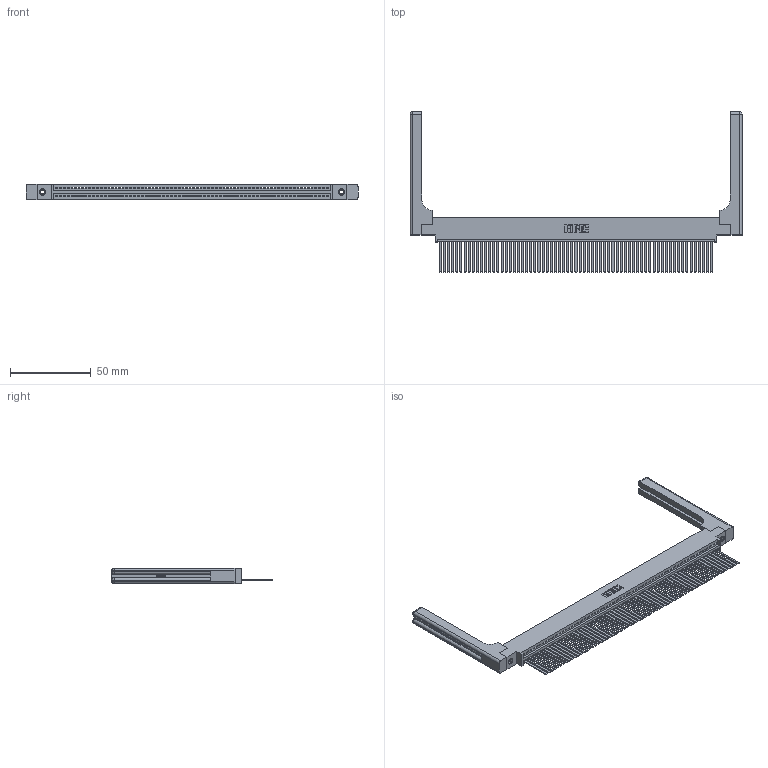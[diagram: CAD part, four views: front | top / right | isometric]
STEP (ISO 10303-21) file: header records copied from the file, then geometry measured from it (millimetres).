
FILE_DESCRIPTION (( 'STEP AP203' ), '1' );
FILE_NAME ('345-067-544-658.STEP', '2019-10-12T03:16:25', ( '' ), ( '' ), 'SwSTEP 2.0', 'SolidWorks 2016', '' );
FILE_SCHEMA (( 'CONFIG_CONTROL_DESIGN' ));
Length unit declared in the file: inch
Products named in the file (5): 345-250-001_345-250-001-102; 345 Part_0.170 Offset - 0.156 Dia-TH; 345-292-001_345-293-144; 345-067-544-658; 345-220-058_345-220-058
Assembly tree (72 placements, depth 2):
  345-067-544-658
    345 Part_0.170 Offset - 0.156 Dia-TH
    345-292-001_345-293-144  x67
    345-250-001_345-250-001-102  x2
    345-220-058_345-220-058  x2
Bounding box: 205.21 x 99.24 x 9.4 mm (x, y, z)
Volume: 28863 mm3; surface area: 35155.4 mm2
Topology: 72 solids, 72 shells, 3870 faces, 11605 edges, 7626 vertices
Faces by surface type: plane 2644, cylinder 1166, bspline 36, cone 12, sphere 8, torus 4
Entity records: 52190 total; most frequent: CARTESIAN_POINT 10010, ORIENTED_EDGE 8808, DIRECTION 7650, EDGE_CURVE 4404, LINE 3916, VECTOR 3916, VERTEX_POINT 2926, AXIS2_PLACEMENT_3D 1867
